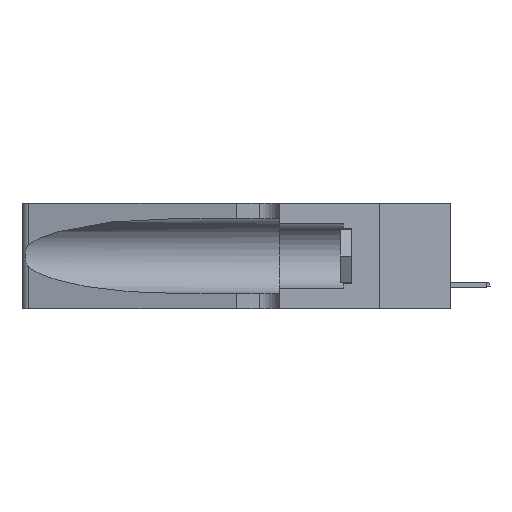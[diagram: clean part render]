
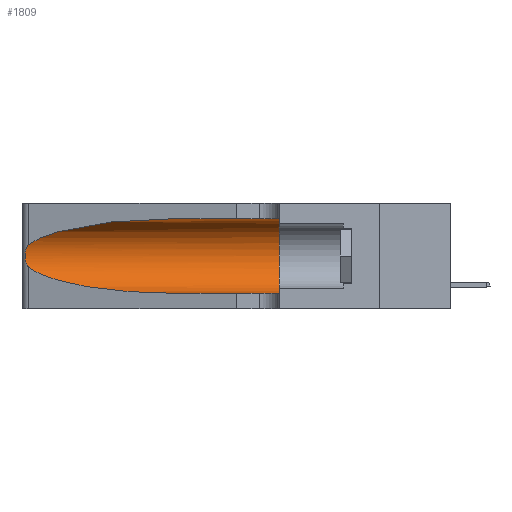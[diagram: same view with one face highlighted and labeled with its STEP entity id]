
A CAD part, left-side view. The second image highlights one B-rep face of the part: STEP entity #1809.
In plain terms, the highlighted cylindrical face has radius 3.308 mm (diameter 6.617 mm), a partial arc.
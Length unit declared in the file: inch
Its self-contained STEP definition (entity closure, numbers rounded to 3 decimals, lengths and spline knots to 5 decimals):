
#46 = CARTESIAN_POINT ( 'NONE',  ( 0.25856, 1.23593, 0.16098 ) ) ;
#466 = VECTOR ( 'NONE', #23796, 39.37008 ) ;
#973 = CARTESIAN_POINT ( 'NONE',  ( 0.1305, 0.72297, 0.05475 ) ) ;
#1809 = ADVANCED_FACE ( 'NONE', ( #21097 ), #4547, .F. ) ;
#2110 = CARTESIAN_POINT ( 'NONE',  ( 0.25787, 1.23484, 0.2124 ) ) ;
#2143 = EDGE_CURVE ( 'NONE', #6146, #6568, #2249, .T. ) ;
#2249 =( BOUNDED_CURVE ( )  B_SPLINE_CURVE ( 3, ( #8275, #14061, #23302, #12015 ),
 .UNSPECIFIED., .F., .T. ) 
 B_SPLINE_CURVE_WITH_KNOTS ( ( 4, 4 ),
 ( 1.5708, 2.84003 ),
 .UNSPECIFIED. ) 
 CURVE ( )  GEOMETRIC_REPRESENTATION_ITEM ( )  RATIONAL_B_SPLINE_CURVE ( ( 1., 0.87, 0.87, 1. ) ) 
 REPRESENTATION_ITEM ( '' )  );
#2340 = VECTOR ( 'NONE', #7619, 39.37008 ) ;
#3238 = EDGE_LOOP ( 'NONE', ( #18690, #18062, #17744, #15366, #18233, #9384 ) ) ;
#3674 = CARTESIAN_POINT ( 'NONE',  ( 0.1305, 1.61858, 0.05475 ) ) ;
#3809 = CARTESIAN_POINT ( 'NONE',  ( 0.25789, 1.23486, 0.15765 ) ) ;
#4547 = CYLINDRICAL_SURFACE ( 'NONE', #7728, 0.13025 ) ;
#5057 = EDGE_CURVE ( 'NONE', #7400, #5233, #13092, .T. ) ;
#5233 = VERTEX_POINT ( 'NONE', #22881 ) ;
#5310 = LINE ( 'NONE', #12678, #2340 ) ;
#5771 = CARTESIAN_POINT ( 'NONE',  ( 0.25487, 1.22718, 0.14631 ) ) ;
#6133 = CARTESIAN_POINT ( 'NONE',  ( 0.25555, 1.22994, 0.2215 ) ) ;
#6146 = VERTEX_POINT ( 'NONE', #12636 ) ;
#6568 = VERTEX_POINT ( 'NONE', #22976 ) ;
#6783 = CARTESIAN_POINT ( 'NONE',  ( 0.2373, 1.15595, 0.08982 ) ) ;
#7400 = VERTEX_POINT ( 'NONE', #973 ) ;
#7492 = B_SPLINE_CURVE_WITH_KNOTS ( 'NONE', 3,
 ( #14922, #6133, #13494, #2110, #20834, #9499, #9238, #18800, #16637, #46, #3809, #9606, #22311, #5771 ),
 .UNSPECIFIED., .F., .F.,
 ( 4, 2, 2, 2, 2, 2, 4 ),
 ( 0., 0.00027, 0.00053, 0.00107, 0.0016, 0.00187, 0.00214 ),
 .UNSPECIFIED. ) ;
#7619 = DIRECTION ( 'NONE',  ( 0., -1., 0. ) ) ;
#7728 = AXIS2_PLACEMENT_3D ( 'NONE', #11922, #8889, #19764 ) ;
#8275 = CARTESIAN_POINT ( 'NONE',  ( 0.1305, 0.72297, 0.31525 ) ) ;
#8889 = DIRECTION ( 'NONE',  ( 0., -1., 0. ) ) ;
#9238 = CARTESIAN_POINT ( 'NONE',  ( 0.26075, 1.23896, 0.19203 ) ) ;
#9384 = ORIENTED_EDGE ( 'NONE', *, *, #18320, .F. ) ;
#9499 = CARTESIAN_POINT ( 'NONE',  ( 0.26018, 1.23835, 0.19895 ) ) ;
#9606 = CARTESIAN_POINT ( 'NONE',  ( 0.25639, 1.23186, 0.15144 ) ) ;
#9643 = CARTESIAN_POINT ( 'NONE',  ( 0.1305, 0.35, 0.31525 ) ) ;
#10143 = CARTESIAN_POINT ( 'NONE',  ( 0.1305, 0.35, 0.185 ) ) ;
#11834 = DIRECTION ( 'NONE',  ( 0., 0., 1. ) ) ;
#11922 = CARTESIAN_POINT ( 'NONE',  ( 0.1305, 1.61858, 0.185 ) ) ;
#11991 =( BOUNDED_CURVE ( )  B_SPLINE_CURVE ( 3, ( #16058, #6783, #15940, #21253 ),
 .UNSPECIFIED., .F., .F. ) 
 B_SPLINE_CURVE_WITH_KNOTS ( ( 4, 4 ),
 ( 3.44316, 4.71239 ),
 .UNSPECIFIED. ) 
 CURVE ( )  GEOMETRIC_REPRESENTATION_ITEM ( )  RATIONAL_B_SPLINE_CURVE ( ( 1., 0.87, 0.87, 1. ) ) 
 REPRESENTATION_ITEM ( '' )  );
#12015 = CARTESIAN_POINT ( 'NONE',  ( 0.25487, 1.22718, 0.22369 ) ) ;
#12636 = CARTESIAN_POINT ( 'NONE',  ( 0.1305, 0.72297, 0.31525 ) ) ;
#12678 = CARTESIAN_POINT ( 'NONE',  ( 0.1305, 1.61858, 0.31525 ) ) ;
#13092 = LINE ( 'NONE', #3674, #466 ) ;
#13376 = CARTESIAN_POINT ( 'NONE',  ( 0.25487, 1.22718, 0.14631 ) ) ;
#13494 = CARTESIAN_POINT ( 'NONE',  ( 0.25639, 1.23184, 0.21858 ) ) ;
#13528 = VERTEX_POINT ( 'NONE', #13376 ) ;
#14061 = CARTESIAN_POINT ( 'NONE',  ( 0.18966, 0.96281, 0.31525 ) ) ;
#14922 = CARTESIAN_POINT ( 'NONE',  ( 0.25487, 1.22718, 0.22369 ) ) ;
#15366 = ORIENTED_EDGE ( 'NONE', *, *, #5057, .T. ) ;
#15761 = AXIS2_PLACEMENT_3D ( 'NONE', #10143, #22869, #11834 ) ;
#15940 = CARTESIAN_POINT ( 'NONE',  ( 0.18966, 0.96281, 0.05475 ) ) ;
#16058 = CARTESIAN_POINT ( 'NONE',  ( 0.25487, 1.22718, 0.14631 ) ) ;
#16637 = CARTESIAN_POINT ( 'NONE',  ( 0.26017, 1.23833, 0.17102 ) ) ;
#17744 = ORIENTED_EDGE ( 'NONE', *, *, #19665, .T. ) ;
#18062 = ORIENTED_EDGE ( 'NONE', *, *, #23871, .T. ) ;
#18233 = ORIENTED_EDGE ( 'NONE', *, *, #23883, .F. ) ;
#18320 = EDGE_CURVE ( 'NONE', #6146, #23339, #5310, .T. ) ;
#18690 = ORIENTED_EDGE ( 'NONE', *, *, #2143, .T. ) ;
#18800 = CARTESIAN_POINT ( 'NONE',  ( 0.26075, 1.23896, 0.178 ) ) ;
#19665 = EDGE_CURVE ( 'NONE', #13528, #7400, #11991, .T. ) ;
#19764 = DIRECTION ( 'NONE',  ( 0., 0., -1. ) ) ;
#20024 = CIRCLE ( 'NONE', #15761, 0.13025 ) ;
#20834 = CARTESIAN_POINT ( 'NONE',  ( 0.25854, 1.2359, 0.20912 ) ) ;
#21097 = FACE_OUTER_BOUND ( 'NONE', #3238, .T. ) ;
#21253 = CARTESIAN_POINT ( 'NONE',  ( 0.1305, 0.72297, 0.05475 ) ) ;
#22311 = CARTESIAN_POINT ( 'NONE',  ( 0.25555, 1.22993, 0.14849 ) ) ;
#22869 = DIRECTION ( 'NONE',  ( 0., 1., 0. ) ) ;
#22881 = CARTESIAN_POINT ( 'NONE',  ( 0.1305, 0.35, 0.05475 ) ) ;
#22976 = CARTESIAN_POINT ( 'NONE',  ( 0.25487, 1.22718, 0.22369 ) ) ;
#23302 = CARTESIAN_POINT ( 'NONE',  ( 0.2373, 1.15595, 0.28018 ) ) ;
#23339 = VERTEX_POINT ( 'NONE', #9643 ) ;
#23796 = DIRECTION ( 'NONE',  ( 0., -1., 0. ) ) ;
#23871 = EDGE_CURVE ( 'NONE', #6568, #13528, #7492, .T. ) ;
#23883 = EDGE_CURVE ( 'NONE', #23339, #5233, #20024, .T. ) ;
